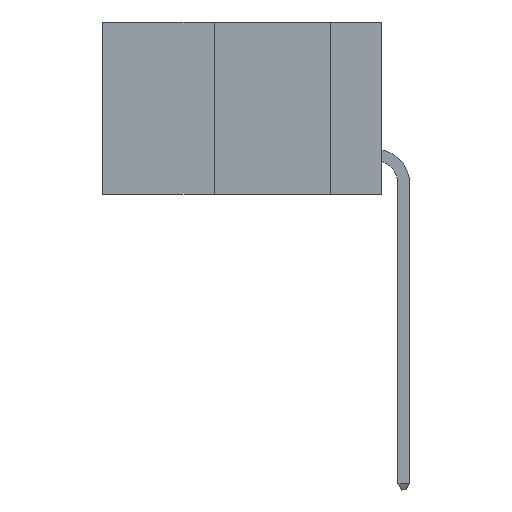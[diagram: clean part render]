
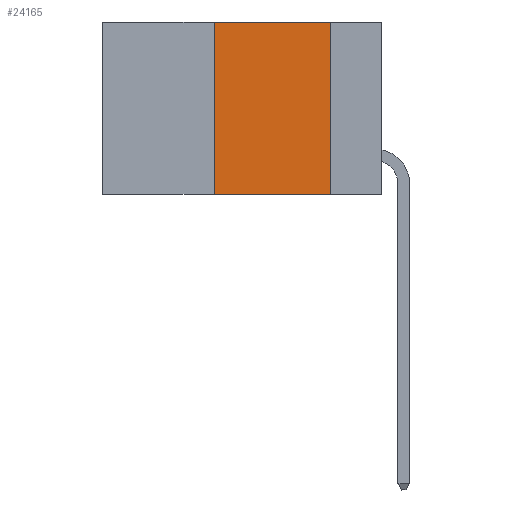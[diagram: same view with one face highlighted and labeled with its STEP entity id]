
A CAD part, left-side view. The second image highlights one B-rep face of the part: STEP entity #24165.
In plain terms, the highlighted planar face has unit normal (-1, 0, 0).
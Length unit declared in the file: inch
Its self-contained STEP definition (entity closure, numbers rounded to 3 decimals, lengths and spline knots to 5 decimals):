
#853 = EDGE_LOOP ( 'NONE', ( #6523, #21585, #20464, #21155 ) ) ;
#975 = DIRECTION ( 'NONE',  ( 0., 0., -1. ) ) ;
#1075 = CARTESIAN_POINT ( 'NONE',  ( 0., 0.6, 0. ) ) ;
#2222 = VERTEX_POINT ( 'NONE', #20030 ) ;
#3205 = VERTEX_POINT ( 'NONE', #21016 ) ;
#3349 = DIRECTION ( 'NONE',  ( 0., -1., 0. ) ) ;
#4784 = VERTEX_POINT ( 'NONE', #6899 ) ;
#5496 = CARTESIAN_POINT ( 'NONE',  ( 0., 0.11, 0. ) ) ;
#5669 = VECTOR ( 'NONE', #25703, 39.37008 ) ;
#6523 = ORIENTED_EDGE ( 'NONE', *, *, #10945, .F. ) ;
#6674 = VECTOR ( 'NONE', #3349, 39.37008 ) ;
#6899 = CARTESIAN_POINT ( 'NONE',  ( 0., 0.36, -0.37 ) ) ;
#7467 = CARTESIAN_POINT ( 'NONE',  ( 0., 0.6, 0. ) ) ;
#10646 = CARTESIAN_POINT ( 'NONE',  ( 0., 0.6, -0.37 ) ) ;
#10945 = EDGE_CURVE ( 'NONE', #2222, #3205, #20110, .T. ) ;
#11210 = VERTEX_POINT ( 'NONE', #26465 ) ;
#11443 = AXIS2_PLACEMENT_3D ( 'NONE', #7467, #16281, #27110 ) ;
#11718 = PLANE ( 'NONE',  #11443 ) ;
#12384 = LINE ( 'NONE', #1075, #6674 ) ;
#12574 = CARTESIAN_POINT ( 'NONE',  ( 0., 0.36, 0. ) ) ;
#13455 = EDGE_CURVE ( 'NONE', #4784, #11210, #16868, .T. ) ;
#16281 = DIRECTION ( 'NONE',  ( 1., 0., 0. ) ) ;
#16868 = LINE ( 'NONE', #12574, #5669 ) ;
#17806 = EDGE_CURVE ( 'NONE', #4784, #3205, #26731, .T. ) ;
#20030 = CARTESIAN_POINT ( 'NONE',  ( 0., 0.11, 0. ) ) ;
#20110 = LINE ( 'NONE', #5496, #24832 ) ;
#20383 = FACE_OUTER_BOUND ( 'NONE', #853, .T. ) ;
#20464 = ORIENTED_EDGE ( 'NONE', *, *, #13455, .F. ) ;
#21016 = CARTESIAN_POINT ( 'NONE',  ( 0., 0.11, -0.37 ) ) ;
#21155 = ORIENTED_EDGE ( 'NONE', *, *, #17806, .T. ) ;
#21585 = ORIENTED_EDGE ( 'NONE', *, *, #27490, .F. ) ;
#22667 = VECTOR ( 'NONE', #27812, 39.37008 ) ;
#24165 = ADVANCED_FACE ( 'NONE', ( #20383 ), #11718, .F. ) ;
#24832 = VECTOR ( 'NONE', #975, 39.37008 ) ;
#25703 = DIRECTION ( 'NONE',  ( 0., 0., 1. ) ) ;
#26465 = CARTESIAN_POINT ( 'NONE',  ( 0., 0.36, 0. ) ) ;
#26731 = LINE ( 'NONE', #10646, #22667 ) ;
#27110 = DIRECTION ( 'NONE',  ( 0., 0., -1. ) ) ;
#27490 = EDGE_CURVE ( 'NONE', #11210, #2222, #12384, .T. ) ;
#27812 = DIRECTION ( 'NONE',  ( 0., -1., 0. ) ) ;
